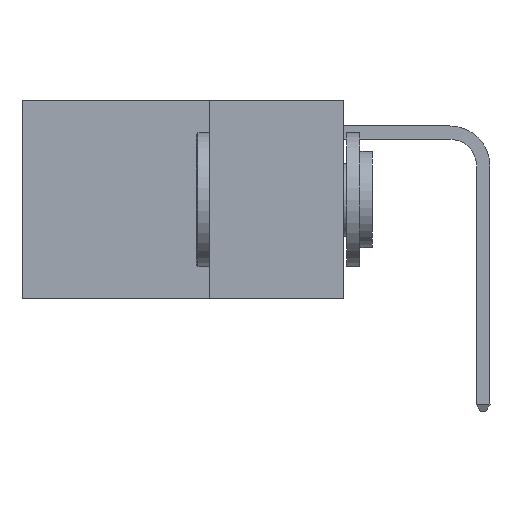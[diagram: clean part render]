
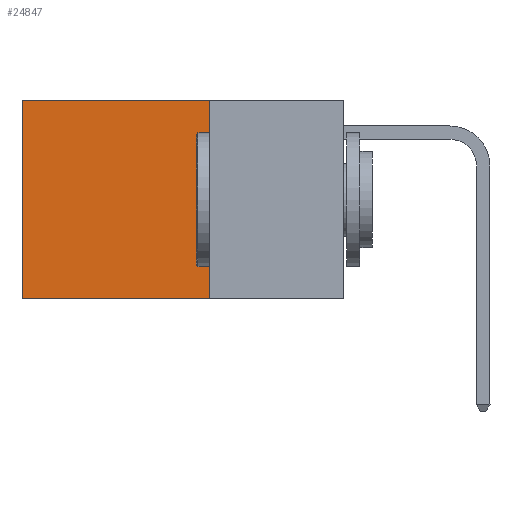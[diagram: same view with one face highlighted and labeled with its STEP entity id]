
A CAD part, left-side view. The second image highlights one B-rep face of the part: STEP entity #24847.
In plain terms, the highlighted planar face has unit normal (-1, 0, 0).
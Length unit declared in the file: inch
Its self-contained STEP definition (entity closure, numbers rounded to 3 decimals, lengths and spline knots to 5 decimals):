
#1082 = VERTEX_POINT ( 'NONE', #9425 ) ;
#2106 = ORIENTED_EDGE ( 'NONE', *, *, #23075, .T. ) ;
#2269 = LINE ( 'NONE', #6263, #11109 ) ;
#2628 = DIRECTION ( 'NONE',  ( 0., 1., 0. ) ) ;
#2724 = DIRECTION ( 'NONE',  ( 0., 0., -1. ) ) ;
#4389 = PLANE ( 'NONE',  #7003 ) ;
#6263 = CARTESIAN_POINT ( 'NONE',  ( 0.2625, 0.25, 0. ) ) ;
#6526 = CARTESIAN_POINT ( 'NONE',  ( 0.2625, 0.25, 0. ) ) ;
#6725 = ORIENTED_EDGE ( 'NONE', *, *, #9416, .T. ) ;
#7003 = AXIS2_PLACEMENT_3D ( 'NONE', #15419, #11140, #11006 ) ;
#7310 = VERTEX_POINT ( 'NONE', #19273 ) ;
#8035 = VERTEX_POINT ( 'NONE', #11239 ) ;
#8588 = LINE ( 'NONE', #6526, #19570 ) ;
#9416 = EDGE_CURVE ( 'NONE', #8035, #7310, #2269, .T. ) ;
#9425 = CARTESIAN_POINT ( 'NONE',  ( 0.2625, 0.25, -0.37 ) ) ;
#10806 = DIRECTION ( 'NONE',  ( 0., 1., 0. ) ) ;
#10898 = VECTOR ( 'NONE', #2628, 39.37008 ) ;
#11006 = DIRECTION ( 'NONE',  ( 0., 0., -1. ) ) ;
#11109 = VECTOR ( 'NONE', #10806, 39.37008 ) ;
#11140 = DIRECTION ( 'NONE',  ( 1., 0., 0. ) ) ;
#11239 = CARTESIAN_POINT ( 'NONE',  ( 0.2625, 0.25, 0. ) ) ;
#11552 = CARTESIAN_POINT ( 'NONE',  ( 0.2625, 0.6, 0. ) ) ;
#13259 = EDGE_CURVE ( 'NONE', #8035, #1082, #8588, .T. ) ;
#15089 = DIRECTION ( 'NONE',  ( 0., 0., -1. ) ) ;
#15419 = CARTESIAN_POINT ( 'NONE',  ( 0.2625, 0.25, 0. ) ) ;
#16098 = CARTESIAN_POINT ( 'NONE',  ( 0.2625, 0.6, -0.37 ) ) ;
#16264 = ORIENTED_EDGE ( 'NONE', *, *, #16702, .F. ) ;
#16702 = EDGE_CURVE ( 'NONE', #1082, #26387, #23446, .T. ) ;
#19273 = CARTESIAN_POINT ( 'NONE',  ( 0.2625, 0.6, 0. ) ) ;
#19570 = VECTOR ( 'NONE', #15089, 39.37008 ) ;
#21381 = CARTESIAN_POINT ( 'NONE',  ( 0.2625, 0.25, -0.37 ) ) ;
#21439 = EDGE_LOOP ( 'NONE', ( #2106, #16264, #26518, #6725 ) ) ;
#21481 = FACE_OUTER_BOUND ( 'NONE', #21439, .T. ) ;
#21614 = LINE ( 'NONE', #11552, #23678 ) ;
#23075 = EDGE_CURVE ( 'NONE', #7310, #26387, #21614, .T. ) ;
#23446 = LINE ( 'NONE', #21381, #10898 ) ;
#23678 = VECTOR ( 'NONE', #2724, 39.37008 ) ;
#24847 = ADVANCED_FACE ( 'NONE', ( #21481 ), #4389, .F. ) ;
#26387 = VERTEX_POINT ( 'NONE', #16098 ) ;
#26518 = ORIENTED_EDGE ( 'NONE', *, *, #13259, .F. ) ;
